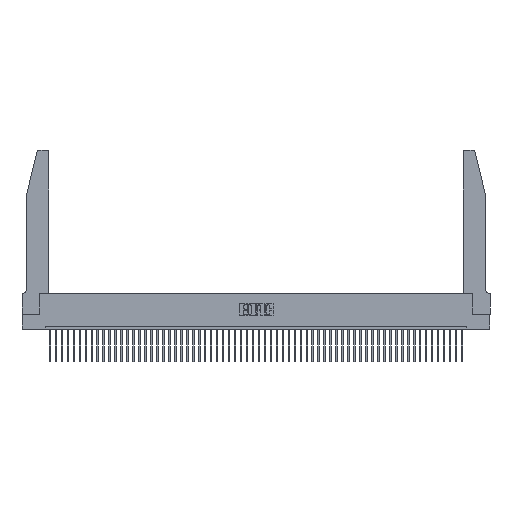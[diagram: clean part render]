
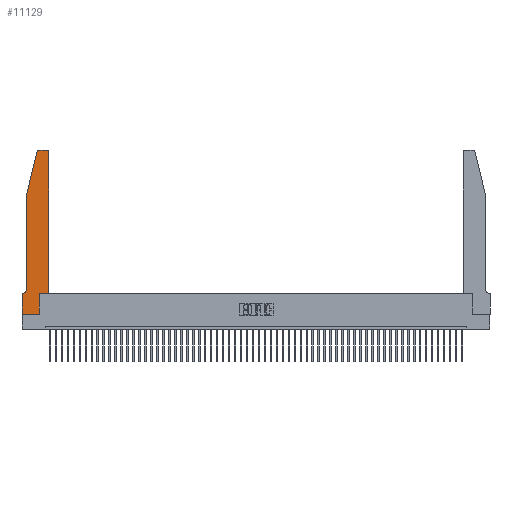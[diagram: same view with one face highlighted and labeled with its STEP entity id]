
A CAD part, top view. The second image highlights one B-rep face of the part: STEP entity #11129.
In plain terms, the highlighted planar face has unit normal (0, 0, 1).
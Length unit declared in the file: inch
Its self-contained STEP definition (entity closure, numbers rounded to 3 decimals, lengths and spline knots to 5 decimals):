
#3473 = CARTESIAN_POINT ( 'NONE',  ( 0.4505, 2.72, 0.37 ) ) ;
#4234 = LINE ( 'NONE', #19197, #39152 ) ;
#5116 = CIRCLE ( 'NONE', #13123, 0.03 ) ;
#5889 = DIRECTION ( 'NONE',  ( 0., 1., 0. ) ) ;
#6146 = ORIENTED_EDGE ( 'NONE', *, *, #49818, .T. ) ;
#6230 = VECTOR ( 'NONE', #17833, 39.37008 ) ;
#8794 = AXIS2_PLACEMENT_3D ( 'NONE', #22830, #27169, #14893 ) ;
#8836 = EDGE_CURVE ( 'NONE', #19025, #13936, #11749, .T. ) ;
#9286 = CARTESIAN_POINT ( 'NONE',  ( 0.2865, 0., 0.37 ) ) ;
#9734 = VECTOR ( 'NONE', #35997, 39.37008 ) ;
#9917 = AXIS2_PLACEMENT_3D ( 'NONE', #11112, #40302, #15520 ) ;
#10758 = DIRECTION ( 'NONE',  ( 1., 0., 0. ) ) ;
#11060 = LINE ( 'NONE', #52506, #9734 ) ;
#11112 = CARTESIAN_POINT ( 'NONE',  ( 0., 0.35, 0.37 ) ) ;
#11129 = ADVANCED_FACE ( 'NONE', ( #52998 ), #23455, .T. ) ;
#11749 = LINE ( 'NONE', #32402, #38921 ) ;
#12499 = VERTEX_POINT ( 'NONE', #53251 ) ;
#12745 = VERTEX_POINT ( 'NONE', #14255 ) ;
#13123 = AXIS2_PLACEMENT_3D ( 'NONE', #30101, #47737, #10758 ) ;
#13894 = CARTESIAN_POINT ( 'NONE',  ( 0., 0., 0.37 ) ) ;
#13936 = VERTEX_POINT ( 'NONE', #49753 ) ;
#14255 = CARTESIAN_POINT ( 'NONE',  ( 0.2865, 0.35, 0.37 ) ) ;
#14710 = EDGE_CURVE ( 'NONE', #38423, #12499, #5116, .T. ) ;
#14893 = DIRECTION ( 'NONE',  ( 1., 0., 0. ) ) ;
#15212 = ORIENTED_EDGE ( 'NONE', *, *, #38998, .T. ) ;
#15520 = DIRECTION ( 'NONE',  ( 1., 0., 0. ) ) ;
#16454 = CARTESIAN_POINT ( 'NONE',  ( 0.2605, 2.75, 0.37 ) ) ;
#16796 = DIRECTION ( 'NONE',  ( -1., 0., 0. ) ) ;
#17364 = VERTEX_POINT ( 'NONE', #9286 ) ;
#17833 = DIRECTION ( 'NONE',  ( 0., 1., 0. ) ) ;
#17884 = EDGE_CURVE ( 'NONE', #38082, #19025, #31309, .T. ) ;
#18751 = ORIENTED_EDGE ( 'NONE', *, *, #29404, .T. ) ;
#18986 = ORIENTED_EDGE ( 'NONE', *, *, #17884, .T. ) ;
#19025 = VERTEX_POINT ( 'NONE', #50389 ) ;
#19197 = CARTESIAN_POINT ( 'NONE',  ( 0.0755, 2., 0.37 ) ) ;
#19552 = DIRECTION ( 'NONE',  ( 0., -1., 0. ) ) ;
#21538 = DIRECTION ( 'NONE',  ( -1., 0., 0. ) ) ;
#21757 = DIRECTION ( 'NONE',  ( 1., 0., 0. ) ) ;
#22549 = CARTESIAN_POINT ( 'NONE',  ( 0.4205, 2.75, 0.37 ) ) ;
#22830 = CARTESIAN_POINT ( 'NONE',  ( 0.4205, 2.72, 0.37 ) ) ;
#22894 = LINE ( 'NONE', #13894, #40453 ) ;
#22923 = LINE ( 'NONE', #16454, #24259 ) ;
#22943 = VECTOR ( 'NONE', #21757, 39.37008 ) ;
#23455 = PLANE ( 'NONE',  #9917 ) ;
#23486 = ORIENTED_EDGE ( 'NONE', *, *, #39761, .T. ) ;
#23693 = AXIS2_PLACEMENT_3D ( 'NONE', #35950, #45510, #21538 ) ;
#24259 = VECTOR ( 'NONE', #16796, 39.37008 ) ;
#25605 = CIRCLE ( 'NONE', #8794, 0.03 ) ;
#25613 = LINE ( 'NONE', #33947, #6230 ) ;
#26381 = VERTEX_POINT ( 'NONE', #22549 ) ;
#26576 = VERTEX_POINT ( 'NONE', #48072 ) ;
#26787 = EDGE_LOOP ( 'NONE', ( #48568, #48977, #39034, #52293, #18986, #49847, #15212, #33902, #52428, #18751, #23486, #6146 ) ) ;
#27169 = DIRECTION ( 'NONE',  ( 0., 0., 1. ) ) ;
#27864 = EDGE_CURVE ( 'NONE', #17364, #12745, #47089, .T. ) ;
#28373 = VERTEX_POINT ( 'NONE', #37386 ) ;
#28553 = VECTOR ( 'NONE', #41882, 39.37008 ) ;
#28572 = DIRECTION ( 'NONE',  ( -1., 0., 0. ) ) ;
#29404 = EDGE_CURVE ( 'NONE', #12745, #53114, #53455, .T. ) ;
#30101 = CARTESIAN_POINT ( 'NONE',  ( 0.284, 2.72, 0.37 ) ) ;
#31309 = CIRCLE ( 'NONE', #23693, 0.07 ) ;
#32402 = CARTESIAN_POINT ( 'NONE',  ( 0.0755, 0.35, 0.37 ) ) ;
#32467 = LINE ( 'NONE', #36173, #28553 ) ;
#33424 = CARTESIAN_POINT ( 'NONE',  ( 0.0755, 0.42, 0.37 ) ) ;
#33902 = ORIENTED_EDGE ( 'NONE', *, *, #37799, .T. ) ;
#33947 = CARTESIAN_POINT ( 'NONE',  ( 0.4505, 0.35, 0.37 ) ) ;
#35950 = CARTESIAN_POINT ( 'NONE',  ( 0.0055, 0.42, 0.37 ) ) ;
#35997 = DIRECTION ( 'NONE',  ( -0.239, -0.971, 0. ) ) ;
#36173 = CARTESIAN_POINT ( 'NONE',  ( 0., 0., 0.37 ) ) ;
#37386 = CARTESIAN_POINT ( 'NONE',  ( 0.0755, 2., 0.37 ) ) ;
#37398 = VECTOR ( 'NONE', #5889, 39.37008 ) ;
#37799 = EDGE_CURVE ( 'NONE', #26576, #17364, #22894, .T. ) ;
#38082 = VERTEX_POINT ( 'NONE', #33424 ) ;
#38423 = VERTEX_POINT ( 'NONE', #51164 ) ;
#38825 = CARTESIAN_POINT ( 'NONE',  ( 0.2865, 0.35, 0.37 ) ) ;
#38921 = VECTOR ( 'NONE', #28572, 39.37008 ) ;
#38972 = CARTESIAN_POINT ( 'NONE',  ( 0.4505, 0.35, 0.37 ) ) ;
#38998 = EDGE_CURVE ( 'NONE', #13936, #26576, #32467, .T. ) ;
#39034 = ORIENTED_EDGE ( 'NONE', *, *, #43146, .T. ) ;
#39152 = VECTOR ( 'NONE', #19552, 39.37008 ) ;
#39470 = EDGE_CURVE ( 'NONE', #28373, #38082, #4234, .T. ) ;
#39761 = EDGE_CURVE ( 'NONE', #53114, #42666, #25613, .T. ) ;
#40302 = DIRECTION ( 'NONE',  ( 0., 0., 1. ) ) ;
#40453 = VECTOR ( 'NONE', #42883, 39.37008 ) ;
#41882 = DIRECTION ( 'NONE',  ( 0., -1., 0. ) ) ;
#42666 = VERTEX_POINT ( 'NONE', #3473 ) ;
#42883 = DIRECTION ( 'NONE',  ( 1., 0., 0. ) ) ;
#43146 = EDGE_CURVE ( 'NONE', #12499, #28373, #11060, .T. ) ;
#45510 = DIRECTION ( 'NONE',  ( 0., 0., -1. ) ) ;
#45668 = CARTESIAN_POINT ( 'NONE',  ( 0.4505, 0.35, 0.37 ) ) ;
#45799 = EDGE_CURVE ( 'NONE', #26381, #38423, #22923, .T. ) ;
#47089 = LINE ( 'NONE', #38825, #37398 ) ;
#47737 = DIRECTION ( 'NONE',  ( 0., 0., 1. ) ) ;
#48072 = CARTESIAN_POINT ( 'NONE',  ( 0., 0., 0.37 ) ) ;
#48568 = ORIENTED_EDGE ( 'NONE', *, *, #45799, .T. ) ;
#48977 = ORIENTED_EDGE ( 'NONE', *, *, #14710, .T. ) ;
#49753 = CARTESIAN_POINT ( 'NONE',  ( 0., 0.35, 0.37 ) ) ;
#49818 = EDGE_CURVE ( 'NONE', #42666, #26381, #25605, .T. ) ;
#49847 = ORIENTED_EDGE ( 'NONE', *, *, #8836, .T. ) ;
#50389 = CARTESIAN_POINT ( 'NONE',  ( 0.0055, 0.35, 0.37 ) ) ;
#51164 = CARTESIAN_POINT ( 'NONE',  ( 0.284, 2.75, 0.37 ) ) ;
#52293 = ORIENTED_EDGE ( 'NONE', *, *, #39470, .T. ) ;
#52428 = ORIENTED_EDGE ( 'NONE', *, *, #27864, .T. ) ;
#52506 = CARTESIAN_POINT ( 'NONE',  ( 0.0755, 2., 0.37 ) ) ;
#52998 = FACE_OUTER_BOUND ( 'NONE', #26787, .T. ) ;
#53114 = VERTEX_POINT ( 'NONE', #45668 ) ;
#53251 = CARTESIAN_POINT ( 'NONE',  ( 0.25487, 2.72718, 0.37 ) ) ;
#53455 = LINE ( 'NONE', #38972, #22943 ) ;
